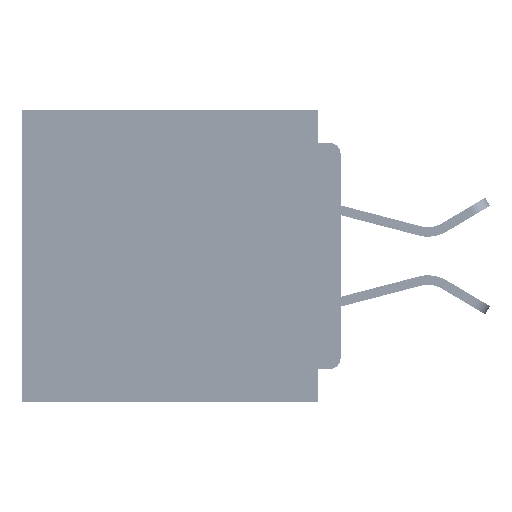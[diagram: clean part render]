
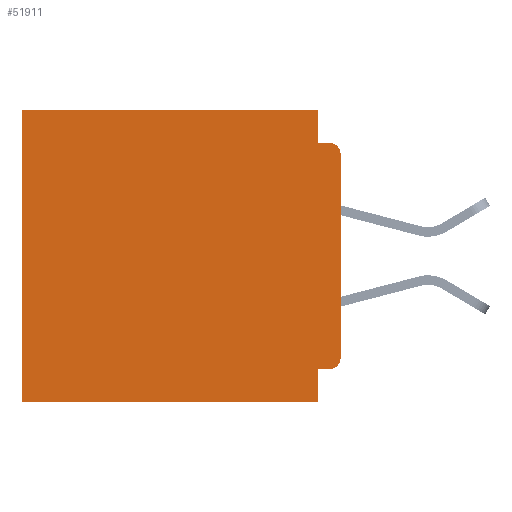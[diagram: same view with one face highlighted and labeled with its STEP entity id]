
A CAD part, left-side view. The second image highlights one B-rep face of the part: STEP entity #51911.
In plain terms, the highlighted planar face has unit normal (-1, 0, 0).
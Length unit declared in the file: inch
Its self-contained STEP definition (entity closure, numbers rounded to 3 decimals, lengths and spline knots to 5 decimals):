
#274 = AXIS2_PLACEMENT_3D ( 'NONE', #36401, #10720, #40668 ) ;
#282 = CARTESIAN_POINT ( 'NONE',  ( 0.3, 0.437, 0. ) ) ;
#600 = CARTESIAN_POINT ( 'NONE',  ( 0.3, 0.031, -0.4 ) ) ;
#1135 = EDGE_CURVE ( 'NONE', #30195, #24753, #24682, .T. ) ;
#1476 = CIRCLE ( 'NONE', #274, 0.015 ) ;
#1873 = VECTOR ( 'NONE', #17687, 39.37008 ) ;
#2257 = ORIENTED_EDGE ( 'NONE', *, *, #14751, .T. ) ;
#2399 = EDGE_CURVE ( 'NONE', #11464, #40662, #48675, .T. ) ;
#2684 = EDGE_CURVE ( 'NONE', #23113, #24638, #23995, .T. ) ;
#3145 = CARTESIAN_POINT ( 'NONE',  ( 0.3, 0.437, -0.4 ) ) ;
#4047 = CARTESIAN_POINT ( 'NONE',  ( 0.3, 0.031, 0. ) ) ;
#5841 = LINE ( 'NONE', #17357, #26012 ) ;
#5844 = AXIS2_PLACEMENT_3D ( 'NONE', #14763, #44646, #19097 ) ;
#6123 = DIRECTION ( 'NONE',  ( 0., -1., 0. ) ) ;
#6959 = CARTESIAN_POINT ( 'NONE',  ( 0.3, 0., -0.4 ) ) ;
#9435 = CARTESIAN_POINT ( 'NONE',  ( 0.3, 0.015, -0.045 ) ) ;
#10720 = DIRECTION ( 'NONE',  ( -1., 0., 0. ) ) ;
#10934 = ORIENTED_EDGE ( 'NONE', *, *, #48245, .F. ) ;
#11216 = VECTOR ( 'NONE', #32939, 39.37008 ) ;
#11279 = DIRECTION ( 'NONE',  ( 0., 0., -1. ) ) ;
#11464 = VERTEX_POINT ( 'NONE', #4047 ) ;
#11555 = ORIENTED_EDGE ( 'NONE', *, *, #45315, .T. ) ;
#11845 = AXIS2_PLACEMENT_3D ( 'NONE', #6959, #36958, #11279 ) ;
#14338 = EDGE_CURVE ( 'NONE', #22446, #24753, #5841, .T. ) ;
#14751 = EDGE_CURVE ( 'NONE', #11464, #30195, #39395, .T. ) ;
#14763 = CARTESIAN_POINT ( 'NONE',  ( 0.3, 0.015, -0.34 ) ) ;
#16426 = DIRECTION ( 'NONE',  ( 0., 1., 0. ) ) ;
#17309 = CARTESIAN_POINT ( 'NONE',  ( 0.3, 0., -0.355 ) ) ;
#17357 = CARTESIAN_POINT ( 'NONE',  ( 0.3, 0., -0.4 ) ) ;
#17687 = DIRECTION ( 'NONE',  ( 0., 0., -1. ) ) ;
#19097 = DIRECTION ( 'NONE',  ( 0., 0., -1. ) ) ;
#20060 = EDGE_CURVE ( 'NONE', #28908, #22446, #54785, .T. ) ;
#20237 = CARTESIAN_POINT ( 'NONE',  ( 0.3, 0., -0.34 ) ) ;
#21045 = VERTEX_POINT ( 'NONE', #9435 ) ;
#22446 = VERTEX_POINT ( 'NONE', #45196 ) ;
#23113 = VERTEX_POINT ( 'NONE', #24237 ) ;
#23881 = ORIENTED_EDGE ( 'NONE', *, *, #2684, .F. ) ;
#23995 = LINE ( 'NONE', #36007, #11216 ) ;
#24064 = PLANE ( 'NONE',  #11845 ) ;
#24184 = EDGE_CURVE ( 'NONE', #46326, #28908, #30708, .T. ) ;
#24237 = CARTESIAN_POINT ( 'NONE',  ( 0.3, 0., -0.06 ) ) ;
#24638 = VERTEX_POINT ( 'NONE', #20237 ) ;
#24682 = LINE ( 'NONE', #3145, #1873 ) ;
#24710 = VECTOR ( 'NONE', #28468, 39.37008 ) ;
#24753 = VERTEX_POINT ( 'NONE', #37983 ) ;
#25702 = CARTESIAN_POINT ( 'NONE',  ( 0.3, 0.031, -0.045 ) ) ;
#26012 = VECTOR ( 'NONE', #30089, 39.37008 ) ;
#26095 = CARTESIAN_POINT ( 'NONE',  ( 0.3, 0.031, -0.355 ) ) ;
#26308 = DIRECTION ( 'NONE',  ( 0., 0., -1. ) ) ;
#27163 = ORIENTED_EDGE ( 'NONE', *, *, #1135, .T. ) ;
#27536 = CARTESIAN_POINT ( 'NONE',  ( 0.3, 0., -0.045 ) ) ;
#28468 = DIRECTION ( 'NONE',  ( 0., 0., -1. ) ) ;
#28908 = VERTEX_POINT ( 'NONE', #26095 ) ;
#29404 = VECTOR ( 'NONE', #16426, 39.37008 ) ;
#29990 = EDGE_LOOP ( 'NONE', ( #23881, #32658, #10934, #52990, #2257, #27163, #40175, #54536, #38638, #11555 ) ) ;
#30089 = DIRECTION ( 'NONE',  ( 0., 1., 0. ) ) ;
#30195 = VERTEX_POINT ( 'NONE', #282 ) ;
#30708 = LINE ( 'NONE', #17309, #50561 ) ;
#32658 = ORIENTED_EDGE ( 'NONE', *, *, #49971, .T. ) ;
#32939 = DIRECTION ( 'NONE',  ( 0., 0., -1. ) ) ;
#34559 = VECTOR ( 'NONE', #6123, 39.37008 ) ;
#36007 = CARTESIAN_POINT ( 'NONE',  ( 0.3, 0., -0.4 ) ) ;
#36401 = CARTESIAN_POINT ( 'NONE',  ( 0.3, 0.015, -0.06 ) ) ;
#36958 = DIRECTION ( 'NONE',  ( 1., 0., 0. ) ) ;
#37983 = CARTESIAN_POINT ( 'NONE',  ( 0.3, 0.437, -0.4 ) ) ;
#38638 = ORIENTED_EDGE ( 'NONE', *, *, #24184, .F. ) ;
#39395 = LINE ( 'NONE', #42001, #29404 ) ;
#40175 = ORIENTED_EDGE ( 'NONE', *, *, #14338, .F. ) ;
#40662 = VERTEX_POINT ( 'NONE', #25702 ) ;
#40668 = DIRECTION ( 'NONE',  ( 0., 0., -1. ) ) ;
#42001 = CARTESIAN_POINT ( 'NONE',  ( 0.3, 0., 0. ) ) ;
#42157 = VECTOR ( 'NONE', #26308, 39.37008 ) ;
#43866 = CARTESIAN_POINT ( 'NONE',  ( 0.3, 0.031, 0. ) ) ;
#44646 = DIRECTION ( 'NONE',  ( -1., 0., 0. ) ) ;
#45196 = CARTESIAN_POINT ( 'NONE',  ( 0.3, 0.031, -0.4 ) ) ;
#45315 = EDGE_CURVE ( 'NONE', #46326, #24638, #52713, .T. ) ;
#45546 = FACE_OUTER_BOUND ( 'NONE', #29990, .T. ) ;
#45817 = LINE ( 'NONE', #27536, #34559 ) ;
#46326 = VERTEX_POINT ( 'NONE', #48236 ) ;
#48236 = CARTESIAN_POINT ( 'NONE',  ( 0.3, 0.015, -0.355 ) ) ;
#48245 = EDGE_CURVE ( 'NONE', #40662, #21045, #45817, .T. ) ;
#48675 = LINE ( 'NONE', #43866, #24710 ) ;
#49971 = EDGE_CURVE ( 'NONE', #23113, #21045, #1476, .T. ) ;
#50561 = VECTOR ( 'NONE', #51360, 39.37008 ) ;
#51360 = DIRECTION ( 'NONE',  ( 0., 1., 0. ) ) ;
#51911 = ADVANCED_FACE ( 'NONE', ( #45546 ), #24064, .F. ) ;
#52713 = CIRCLE ( 'NONE', #5844, 0.015 ) ;
#52990 = ORIENTED_EDGE ( 'NONE', *, *, #2399, .F. ) ;
#54536 = ORIENTED_EDGE ( 'NONE', *, *, #20060, .F. ) ;
#54785 = LINE ( 'NONE', #600, #42157 ) ;
